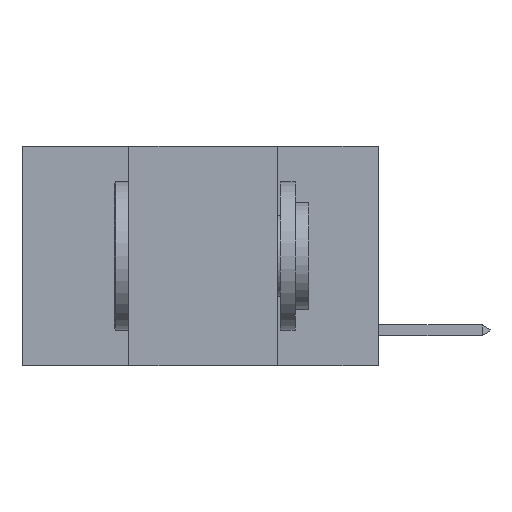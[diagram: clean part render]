
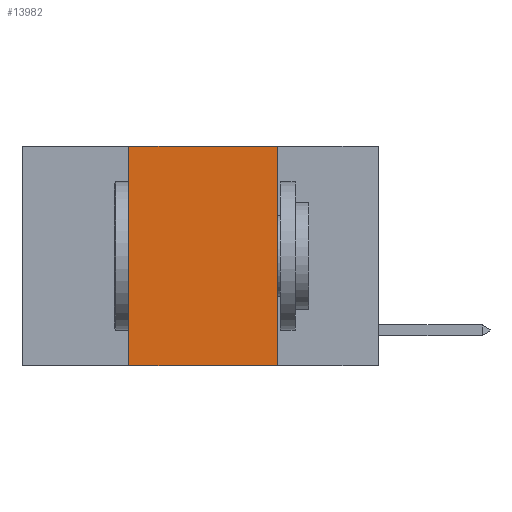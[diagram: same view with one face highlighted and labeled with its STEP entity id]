
A CAD part, left-side view. The second image highlights one B-rep face of the part: STEP entity #13982.
In plain terms, the highlighted planar face has unit normal (-1, 0, 0).
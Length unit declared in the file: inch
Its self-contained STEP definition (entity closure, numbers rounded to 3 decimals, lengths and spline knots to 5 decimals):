
#25 = PLANE ( 'NONE',  #1815 ) ;
#742 = VERTEX_POINT ( 'NONE', #15308 ) ;
#867 = VERTEX_POINT ( 'NONE', #10435 ) ;
#870 = EDGE_CURVE ( 'NONE', #1016, #742, #7065, .T. ) ;
#1016 = VERTEX_POINT ( 'NONE', #7921 ) ;
#1815 = AXIS2_PLACEMENT_3D ( 'NONE', #8490, #13753, #18908 ) ;
#1899 = CARTESIAN_POINT ( 'NONE',  ( 0., 0.6, -0.37 ) ) ;
#3490 = VECTOR ( 'NONE', #21676, 39.37008 ) ;
#3571 = LINE ( 'NONE', #1899, #19685 ) ;
#3775 = ORIENTED_EDGE ( 'NONE', *, *, #7129, .F. ) ;
#5044 = EDGE_CURVE ( 'NONE', #742, #19181, #6094, .T. ) ;
#6094 = LINE ( 'NONE', #12928, #6798 ) ;
#6798 = VECTOR ( 'NONE', #8097, 39.37008 ) ;
#7065 = LINE ( 'NONE', #22046, #16840 ) ;
#7129 = EDGE_CURVE ( 'NONE', #19181, #867, #13089, .T. ) ;
#7921 = CARTESIAN_POINT ( 'NONE',  ( 0., 0.42, -0.37 ) ) ;
#8097 = DIRECTION ( 'NONE',  ( 0., -1., 0. ) ) ;
#8490 = CARTESIAN_POINT ( 'NONE',  ( 0., 0.6, 0. ) ) ;
#10435 = CARTESIAN_POINT ( 'NONE',  ( 0., 0.17, -0.37 ) ) ;
#10815 = ORIENTED_EDGE ( 'NONE', *, *, #19117, .T. ) ;
#12791 = ORIENTED_EDGE ( 'NONE', *, *, #5044, .F. ) ;
#12928 = CARTESIAN_POINT ( 'NONE',  ( 0., 0.6, 0. ) ) ;
#13089 = LINE ( 'NONE', #20027, #3490 ) ;
#13753 = DIRECTION ( 'NONE',  ( 1., 0., 0. ) ) ;
#13861 = FACE_OUTER_BOUND ( 'NONE', #20047, .T. ) ;
#13982 = ADVANCED_FACE ( 'NONE', ( #13861 ), #25, .F. ) ;
#15308 = CARTESIAN_POINT ( 'NONE',  ( 0., 0.42, 0. ) ) ;
#16840 = VECTOR ( 'NONE', #20497, 39.37008 ) ;
#18908 = DIRECTION ( 'NONE',  ( 0., 0., -1. ) ) ;
#19102 = DIRECTION ( 'NONE',  ( 0., -1., 0. ) ) ;
#19117 = EDGE_CURVE ( 'NONE', #1016, #867, #3571, .T. ) ;
#19181 = VERTEX_POINT ( 'NONE', #21664 ) ;
#19685 = VECTOR ( 'NONE', #19102, 39.37008 ) ;
#20027 = CARTESIAN_POINT ( 'NONE',  ( 0., 0.17, 0. ) ) ;
#20047 = EDGE_LOOP ( 'NONE', ( #3775, #12791, #20464, #10815 ) ) ;
#20464 = ORIENTED_EDGE ( 'NONE', *, *, #870, .F. ) ;
#20497 = DIRECTION ( 'NONE',  ( 0., 0., 1. ) ) ;
#21664 = CARTESIAN_POINT ( 'NONE',  ( 0., 0.17, 0. ) ) ;
#21676 = DIRECTION ( 'NONE',  ( 0., 0., -1. ) ) ;
#22046 = CARTESIAN_POINT ( 'NONE',  ( 0., 0.42, 0. ) ) ;
